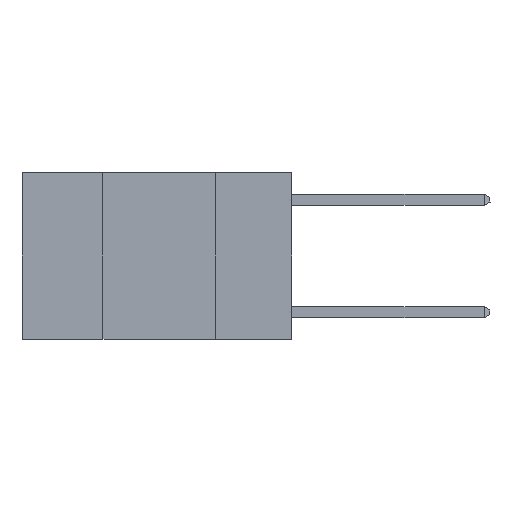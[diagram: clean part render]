
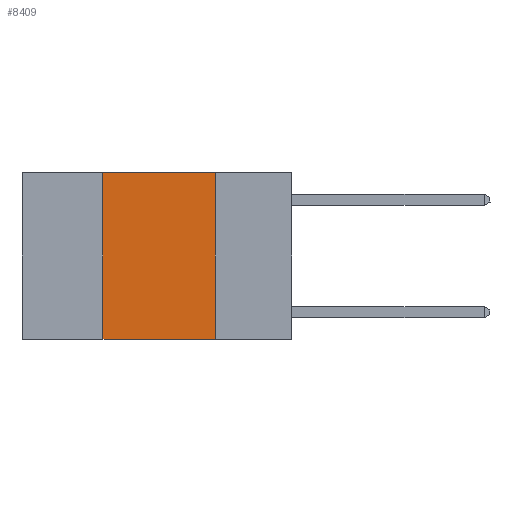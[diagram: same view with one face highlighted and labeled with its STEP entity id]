
A CAD part, left-side view. The second image highlights one B-rep face of the part: STEP entity #8409.
In plain terms, the highlighted planar face has unit normal (-1, 0, 0).
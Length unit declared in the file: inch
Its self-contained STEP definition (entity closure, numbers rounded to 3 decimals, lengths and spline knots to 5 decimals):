
#461 = EDGE_CURVE ( 'NONE', #8709, #6506, #15089, .T. ) ;
#633 = DIRECTION ( 'NONE',  ( 1., 0., 0. ) ) ;
#739 = LINE ( 'NONE', #12837, #3567 ) ;
#1155 = CARTESIAN_POINT ( 'NONE',  ( 0., 0.42, -0.37 ) ) ;
#1972 = CARTESIAN_POINT ( 'NONE',  ( 0., 0.6, -0.37 ) ) ;
#2240 = ORIENTED_EDGE ( 'NONE', *, *, #9813, .F. ) ;
#2399 = VECTOR ( 'NONE', #10880, 39.37008 ) ;
#3068 = CARTESIAN_POINT ( 'NONE',  ( 0., 0.42, 0. ) ) ;
#3101 = LINE ( 'NONE', #1972, #6310 ) ;
#3567 = VECTOR ( 'NONE', #10369, 39.37008 ) ;
#4715 = ORIENTED_EDGE ( 'NONE', *, *, #11507, .F. ) ;
#4783 = DIRECTION ( 'NONE',  ( 0., 0., 1. ) ) ;
#4801 = CARTESIAN_POINT ( 'NONE',  ( 0., 0.42, 0. ) ) ;
#6259 = AXIS2_PLACEMENT_3D ( 'NONE', #12714, #633, #9035 ) ;
#6310 = VECTOR ( 'NONE', #15283, 39.37008 ) ;
#6506 = VERTEX_POINT ( 'NONE', #3068 ) ;
#8409 = ADVANCED_FACE ( 'NONE', ( #12744 ), #13920, .F. ) ;
#8439 = VERTEX_POINT ( 'NONE', #10303 ) ;
#8677 = ORIENTED_EDGE ( 'NONE', *, *, #461, .F. ) ;
#8709 = VERTEX_POINT ( 'NONE', #1155 ) ;
#9035 = DIRECTION ( 'NONE',  ( 0., 0., -1. ) ) ;
#9049 = EDGE_LOOP ( 'NONE', ( #4715, #2240, #8677, #13464 ) ) ;
#9813 = EDGE_CURVE ( 'NONE', #6506, #8439, #739, .T. ) ;
#10303 = CARTESIAN_POINT ( 'NONE',  ( 0., 0.17, 0. ) ) ;
#10369 = DIRECTION ( 'NONE',  ( 0., -1., 0. ) ) ;
#10824 = CARTESIAN_POINT ( 'NONE',  ( 0., 0.17, -0.37 ) ) ;
#10880 = DIRECTION ( 'NONE',  ( 0., 0., -1. ) ) ;
#11507 = EDGE_CURVE ( 'NONE', #8439, #15271, #12077, .T. ) ;
#11860 = VECTOR ( 'NONE', #4783, 39.37008 ) ;
#12077 = LINE ( 'NONE', #13380, #2399 ) ;
#12714 = CARTESIAN_POINT ( 'NONE',  ( 0., 0.6, 0. ) ) ;
#12744 = FACE_OUTER_BOUND ( 'NONE', #9049, .T. ) ;
#12837 = CARTESIAN_POINT ( 'NONE',  ( 0., 0.6, 0. ) ) ;
#13380 = CARTESIAN_POINT ( 'NONE',  ( 0., 0.17, 0. ) ) ;
#13464 = ORIENTED_EDGE ( 'NONE', *, *, #13657, .T. ) ;
#13657 = EDGE_CURVE ( 'NONE', #8709, #15271, #3101, .T. ) ;
#13920 = PLANE ( 'NONE',  #6259 ) ;
#15089 = LINE ( 'NONE', #4801, #11860 ) ;
#15271 = VERTEX_POINT ( 'NONE', #10824 ) ;
#15283 = DIRECTION ( 'NONE',  ( 0., -1., 0. ) ) ;
